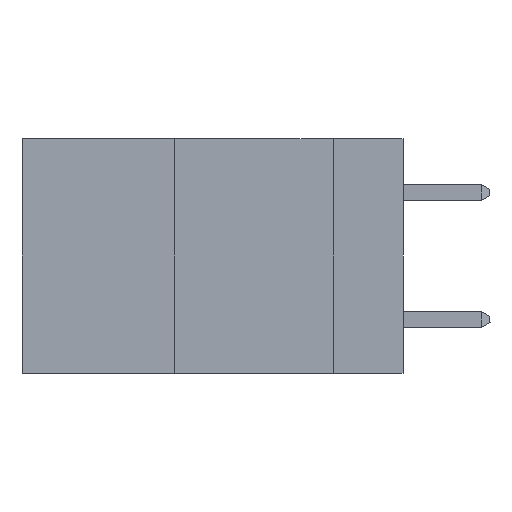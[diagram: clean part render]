
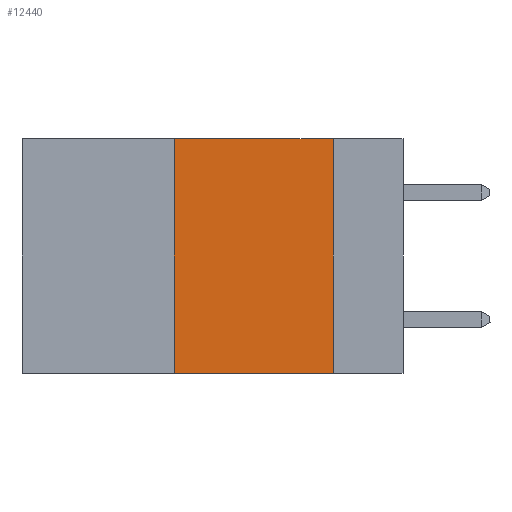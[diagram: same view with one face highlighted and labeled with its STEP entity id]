
A CAD part, left-side view. The second image highlights one B-rep face of the part: STEP entity #12440.
In plain terms, the highlighted planar face has unit normal (-1, 0, 0).
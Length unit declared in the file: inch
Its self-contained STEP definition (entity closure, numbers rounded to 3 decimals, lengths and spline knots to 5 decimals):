
#1215 = EDGE_CURVE ( 'NONE', #20502, #2471, #1829, .T. ) ;
#1829 = LINE ( 'NONE', #15625, #18730 ) ;
#2471 = VERTEX_POINT ( 'NONE', #20451 ) ;
#2825 = DIRECTION ( 'NONE',  ( 0., 0., -1. ) ) ;
#3544 = VECTOR ( 'NONE', #13960, 39.37008 ) ;
#3699 = CARTESIAN_POINT ( 'NONE',  ( 0., 0.11, 0. ) ) ;
#5690 = PLANE ( 'NONE',  #14013 ) ;
#6025 = EDGE_LOOP ( 'NONE', ( #14541, #16557, #18513, #18762 ) ) ;
#7370 = CARTESIAN_POINT ( 'NONE',  ( 0., 0.6, 0. ) ) ;
#8038 = EDGE_CURVE ( 'NONE', #8900, #11244, #21599, .T. ) ;
#8509 = EDGE_CURVE ( 'NONE', #20502, #11244, #21052, .T. ) ;
#8827 = CARTESIAN_POINT ( 'NONE',  ( 0., 0.6, 0. ) ) ;
#8900 = VERTEX_POINT ( 'NONE', #3699 ) ;
#9060 = DIRECTION ( 'NONE',  ( 0., 0., -1. ) ) ;
#9429 = DIRECTION ( 'NONE',  ( 0., -1., 0. ) ) ;
#11244 = VERTEX_POINT ( 'NONE', #15400 ) ;
#12440 = ADVANCED_FACE ( 'NONE', ( #13737 ), #5690, .F. ) ;
#13737 = FACE_OUTER_BOUND ( 'NONE', #6025, .T. ) ;
#13960 = DIRECTION ( 'NONE',  ( 0., -1., 0. ) ) ;
#14013 = AXIS2_PLACEMENT_3D ( 'NONE', #7370, #19123, #9060 ) ;
#14541 = ORIENTED_EDGE ( 'NONE', *, *, #8038, .F. ) ;
#14577 = DIRECTION ( 'NONE',  ( 0., 0., 1. ) ) ;
#15400 = CARTESIAN_POINT ( 'NONE',  ( 0., 0.11, -0.37 ) ) ;
#15625 = CARTESIAN_POINT ( 'NONE',  ( 0., 0.36, 0. ) ) ;
#16557 = ORIENTED_EDGE ( 'NONE', *, *, #21044, .F. ) ;
#16593 = VECTOR ( 'NONE', #9429, 39.37008 ) ;
#17001 = LINE ( 'NONE', #8827, #3544 ) ;
#17148 = VECTOR ( 'NONE', #2825, 39.37008 ) ;
#18513 = ORIENTED_EDGE ( 'NONE', *, *, #1215, .F. ) ;
#18730 = VECTOR ( 'NONE', #14577, 39.37008 ) ;
#18762 = ORIENTED_EDGE ( 'NONE', *, *, #8509, .T. ) ;
#19123 = DIRECTION ( 'NONE',  ( 1., 0., 0. ) ) ;
#19487 = CARTESIAN_POINT ( 'NONE',  ( 0., 0.6, -0.37 ) ) ;
#20451 = CARTESIAN_POINT ( 'NONE',  ( 0., 0.36, 0. ) ) ;
#20502 = VERTEX_POINT ( 'NONE', #20968 ) ;
#20968 = CARTESIAN_POINT ( 'NONE',  ( 0., 0.36, -0.37 ) ) ;
#21044 = EDGE_CURVE ( 'NONE', #2471, #8900, #17001, .T. ) ;
#21052 = LINE ( 'NONE', #19487, #16593 ) ;
#21329 = CARTESIAN_POINT ( 'NONE',  ( 0., 0.11, 0. ) ) ;
#21599 = LINE ( 'NONE', #21329, #17148 ) ;
